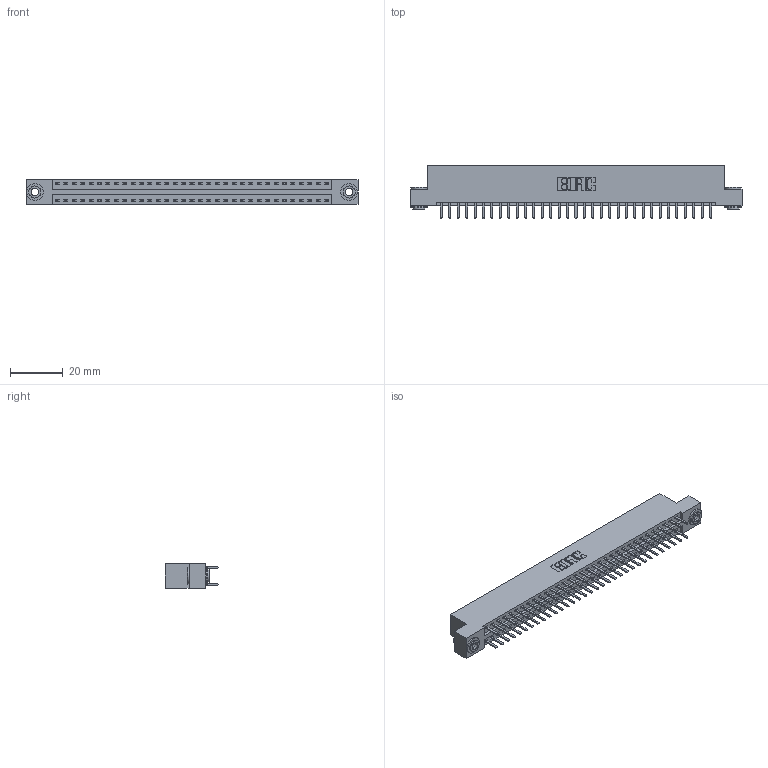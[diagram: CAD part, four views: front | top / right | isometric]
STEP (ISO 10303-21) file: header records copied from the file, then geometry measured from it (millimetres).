
FILE_DESCRIPTION (( 'STEP AP203' ), '1' );
FILE_NAME ('346-066-520-203.STEP', '2022-05-24T16:37:43', ( '' ), ( '' ), 'SwSTEP 2.0', 'SolidWorks 2020', '' );
FILE_SCHEMA (( 'CONFIG_CONTROL_DESIGN' ));
Length unit declared in the file: inch
Products named in the file (4): 346 Part_Flush Mounting Lugs - 0.156 Dia-TH; 345-250-002_345-250-002-102; 345-292-001_345-293-120; 346-066-520-203
Assembly tree (69 placements, depth 2):
  346-066-520-203
    346 Part_Flush Mounting Lugs - 0.156 Dia-TH
    345-292-001_345-293-120  x66
    345-250-002_345-250-002-102  x2
Bounding box: 125.35 x 20.02 x 9.4 mm (x, y, z)
Volume: 12125.5 mm3; surface area: 16706.6 mm2
Topology: 69 solids, 69 shells, 3870 faces, 11199 edges, 7286 vertices
Faces by surface type: plane 2542, cylinder 1320, cone 8
Entity records: 23928 total; most frequent: CARTESIAN_POINT 3949, ORIENTED_EDGE 3862, DIRECTION 3549, EDGE_CURVE 1931, LINE 1639, VECTOR 1639, VERTEX_POINT 1282, AXIS2_PLACEMENT_3D 955
